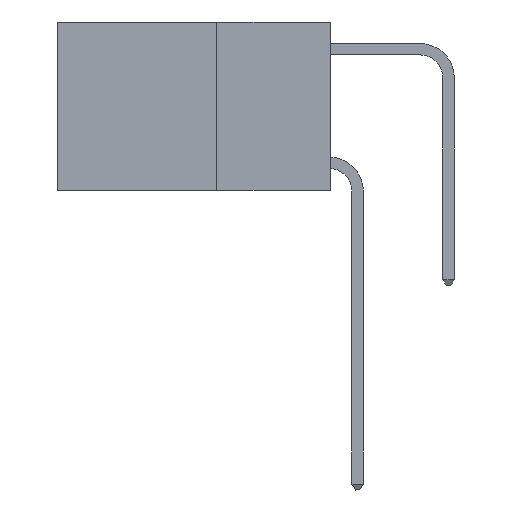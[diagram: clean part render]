
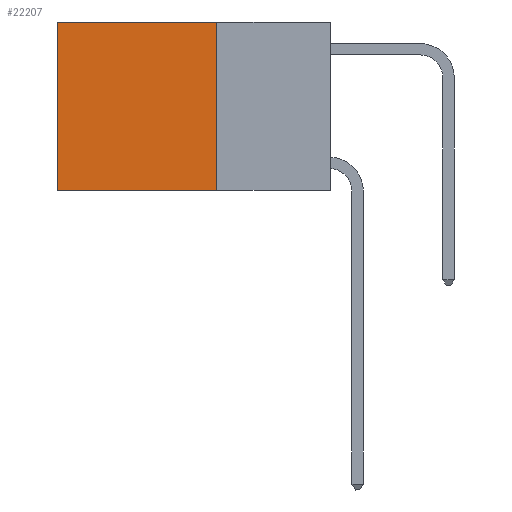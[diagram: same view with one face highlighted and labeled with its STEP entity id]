
A CAD part, left-side view. The second image highlights one B-rep face of the part: STEP entity #22207.
In plain terms, the highlighted planar face has unit normal (-1, 0, 0).
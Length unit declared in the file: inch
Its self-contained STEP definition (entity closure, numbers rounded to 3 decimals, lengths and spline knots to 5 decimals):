
#283 = VERTEX_POINT ( 'NONE', #3988 ) ;
#763 = ORIENTED_EDGE ( 'NONE', *, *, #18915, .F. ) ;
#2971 = LINE ( 'NONE', #22229, #10937 ) ;
#3310 = DIRECTION ( 'NONE',  ( 0., 0., -1. ) ) ;
#3500 = CARTESIAN_POINT ( 'NONE',  ( 0.2625, 0.25, -0.37 ) ) ;
#3609 = LINE ( 'NONE', #3500, #22513 ) ;
#3948 = DIRECTION ( 'NONE',  ( 0., 0., -1. ) ) ;
#3988 = CARTESIAN_POINT ( 'NONE',  ( 0.2625, 0.25, 0. ) ) ;
#4393 = LINE ( 'NONE', #11389, #20304 ) ;
#4846 = VERTEX_POINT ( 'NONE', #17194 ) ;
#5049 = VECTOR ( 'NONE', #5920, 39.37008 ) ;
#5920 = DIRECTION ( 'NONE',  ( 0., 1., 0. ) ) ;
#9084 = ORIENTED_EDGE ( 'NONE', *, *, #18473, .F. ) ;
#9312 = EDGE_CURVE ( 'NONE', #283, #4846, #9377, .T. ) ;
#9353 = CARTESIAN_POINT ( 'NONE',  ( 0.2625, 0.25, 0. ) ) ;
#9377 = LINE ( 'NONE', #16351, #5049 ) ;
#10239 = VERTEX_POINT ( 'NONE', #11341 ) ;
#10358 = EDGE_CURVE ( 'NONE', #4846, #10239, #2971, .T. ) ;
#10633 = ORIENTED_EDGE ( 'NONE', *, *, #9312, .T. ) ;
#10937 = VECTOR ( 'NONE', #3310, 39.37008 ) ;
#11341 = CARTESIAN_POINT ( 'NONE',  ( 0.2625, 0.6, -0.37 ) ) ;
#11389 = CARTESIAN_POINT ( 'NONE',  ( 0.2625, 0.25, 0. ) ) ;
#12776 = PLANE ( 'NONE',  #22312 ) ;
#14487 = DIRECTION ( 'NONE',  ( 1., 0., 0. ) ) ;
#15636 = DIRECTION ( 'NONE',  ( 0., 1., 0. ) ) ;
#16351 = CARTESIAN_POINT ( 'NONE',  ( 0.2625, 0.25, 0. ) ) ;
#16357 = EDGE_LOOP ( 'NONE', ( #20890, #9084, #763, #10633 ) ) ;
#16368 = CARTESIAN_POINT ( 'NONE',  ( 0.2625, 0.25, -0.37 ) ) ;
#17194 = CARTESIAN_POINT ( 'NONE',  ( 0.2625, 0.6, 0. ) ) ;
#17793 = VERTEX_POINT ( 'NONE', #16368 ) ;
#18473 = EDGE_CURVE ( 'NONE', #17793, #10239, #3609, .T. ) ;
#18915 = EDGE_CURVE ( 'NONE', #283, #17793, #4393, .T. ) ;
#19871 = FACE_OUTER_BOUND ( 'NONE', #16357, .T. ) ;
#20304 = VECTOR ( 'NONE', #21938, 39.37008 ) ;
#20890 = ORIENTED_EDGE ( 'NONE', *, *, #10358, .T. ) ;
#21938 = DIRECTION ( 'NONE',  ( 0., 0., -1. ) ) ;
#22207 = ADVANCED_FACE ( 'NONE', ( #19871 ), #12776, .F. ) ;
#22229 = CARTESIAN_POINT ( 'NONE',  ( 0.2625, 0.6, 0. ) ) ;
#22312 = AXIS2_PLACEMENT_3D ( 'NONE', #9353, #14487, #3948 ) ;
#22513 = VECTOR ( 'NONE', #15636, 39.37008 ) ;
